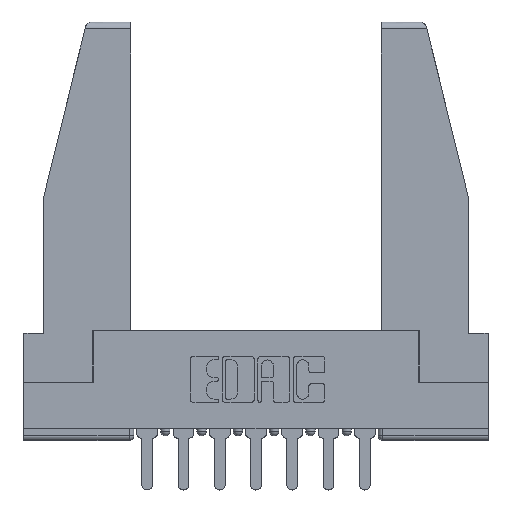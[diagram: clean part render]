
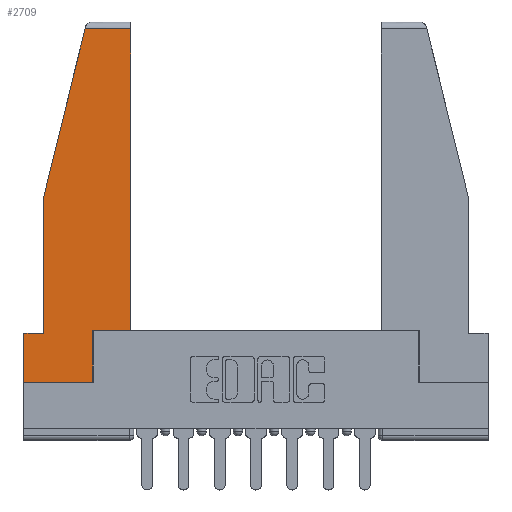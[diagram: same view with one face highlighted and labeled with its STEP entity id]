
A CAD part, top view. The second image highlights one B-rep face of the part: STEP entity #2709.
In plain terms, the highlighted planar face has unit normal (0, 0, 1).
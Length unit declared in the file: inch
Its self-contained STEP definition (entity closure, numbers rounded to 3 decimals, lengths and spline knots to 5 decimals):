
#159 = DIRECTION ( 'NONE',  ( 1., 0., 0. ) ) ;
#207 = VERTEX_POINT ( 'NONE', #12697 ) ;
#845 = VECTOR ( 'NONE', #4236, 39.37008 ) ;
#994 = DIRECTION ( 'NONE',  ( 0., 1., 0. ) ) ;
#996 = DIRECTION ( 'NONE',  ( 0., 1., 0. ) ) ;
#1153 = VERTEX_POINT ( 'NONE', #11010 ) ;
#1228 = DIRECTION ( 'NONE',  ( 1., 0., 0. ) ) ;
#1569 = VECTOR ( 'NONE', #996, 39.37008 ) ;
#1634 = EDGE_CURVE ( 'NONE', #11251, #4211, #3159, .T. ) ;
#1662 = CARTESIAN_POINT ( 'NONE',  ( 0., 1.52, 0. ) ) ;
#1704 = CARTESIAN_POINT ( 'NONE',  ( 0.461, 0.223, 0. ) ) ;
#1830 = EDGE_CURVE ( 'NONE', #12103, #9312, #5680, .T. ) ;
#1930 = EDGE_CURVE ( 'NONE', #4211, #1153, #8738, .T. ) ;
#2596 = VERTEX_POINT ( 'NONE', #8861 ) ;
#2684 = FACE_OUTER_BOUND ( 'NONE', #5577, .T. ) ;
#2698 = ORIENTED_EDGE ( 'NONE', *, *, #1930, .T. ) ;
#2709 = ADVANCED_FACE ( 'NONE', ( #2684 ), #6160, .T. ) ;
#2890 = VECTOR ( 'NONE', #8896, 39.37008 ) ;
#3142 = ORIENTED_EDGE ( 'NONE', *, *, #4959, .T. ) ;
#3159 = LINE ( 'NONE', #6031, #1569 ) ;
#4101 = CARTESIAN_POINT ( 'NONE',  ( 0.086, 0.8, 0. ) ) ;
#4175 = CARTESIAN_POINT ( 'NONE',  ( 0.297, 0., 0. ) ) ;
#4211 = VERTEX_POINT ( 'NONE', #11756 ) ;
#4228 = CARTESIAN_POINT ( 'NONE',  ( 0., 0., 0. ) ) ;
#4236 = DIRECTION ( 'NONE',  ( 0., -1., 0. ) ) ;
#4328 = LINE ( 'NONE', #9168, #845 ) ;
#4407 = DIRECTION ( 'NONE',  ( 0., -1., 0. ) ) ;
#4565 = ORIENTED_EDGE ( 'NONE', *, *, #12896, .T. ) ;
#4702 = ORIENTED_EDGE ( 'NONE', *, *, #1634, .T. ) ;
#4740 = DIRECTION ( 'NONE',  ( -1., 0., 0. ) ) ;
#4813 = DIRECTION ( 'NONE',  ( -1., 0., 0. ) ) ;
#4959 = EDGE_CURVE ( 'NONE', #9312, #5747, #9187, .T. ) ;
#5338 = DIRECTION ( 'NONE',  ( -0.239, -0.971, 0. ) ) ;
#5577 = EDGE_LOOP ( 'NONE', ( #4702, #2698, #4565, #7141, #3142, #5642, #7435, #6879, #11157 ) ) ;
#5642 = ORIENTED_EDGE ( 'NONE', *, *, #6456, .T. ) ;
#5680 = LINE ( 'NONE', #6503, #7847 ) ;
#5747 = VERTEX_POINT ( 'NONE', #12834 ) ;
#5816 = CARTESIAN_POINT ( 'NONE',  ( 0., 0., 0. ) ) ;
#5894 = LINE ( 'NONE', #5816, #2890 ) ;
#6031 = CARTESIAN_POINT ( 'NONE',  ( 0.461, 0.223, 0. ) ) ;
#6160 = PLANE ( 'NONE',  #7338 ) ;
#6456 = EDGE_CURVE ( 'NONE', #5747, #207, #4328, .T. ) ;
#6503 = CARTESIAN_POINT ( 'NONE',  ( 0.086, 0.8, 0. ) ) ;
#6513 = EDGE_CURVE ( 'NONE', #2596, #11251, #12751, .T. ) ;
#6879 = ORIENTED_EDGE ( 'NONE', *, *, #10868, .T. ) ;
#6957 = EDGE_CURVE ( 'NONE', #207, #8160, #5894, .T. ) ;
#7118 = DIRECTION ( 'NONE',  ( 0., 0., 1. ) ) ;
#7141 = ORIENTED_EDGE ( 'NONE', *, *, #1830, .T. ) ;
#7338 = AXIS2_PLACEMENT_3D ( 'NONE', #4228, #7118, #159 ) ;
#7435 = ORIENTED_EDGE ( 'NONE', *, *, #6957, .T. ) ;
#7847 = VECTOR ( 'NONE', #4407, 39.37008 ) ;
#7999 = VECTOR ( 'NONE', #5338, 39.37008 ) ;
#8160 = VERTEX_POINT ( 'NONE', #4175 ) ;
#8314 = VECTOR ( 'NONE', #994, 39.37008 ) ;
#8559 = CARTESIAN_POINT ( 'NONE',  ( 0., 0.21, 0. ) ) ;
#8738 = LINE ( 'NONE', #1662, #10297 ) ;
#8861 = CARTESIAN_POINT ( 'NONE',  ( 0.297, 0.223, 0. ) ) ;
#8896 = DIRECTION ( 'NONE',  ( 1., 0., 0. ) ) ;
#9168 = CARTESIAN_POINT ( 'NONE',  ( 0., 0.21, 0. ) ) ;
#9187 = LINE ( 'NONE', #8559, #10745 ) ;
#9312 = VERTEX_POINT ( 'NONE', #10931 ) ;
#10297 = VECTOR ( 'NONE', #4813, 39.37008 ) ;
#10658 = LINE ( 'NONE', #12114, #8314 ) ;
#10745 = VECTOR ( 'NONE', #4740, 39.37008 ) ;
#10868 = EDGE_CURVE ( 'NONE', #8160, #2596, #10658, .T. ) ;
#10931 = CARTESIAN_POINT ( 'NONE',  ( 0.086, 0.21, 0. ) ) ;
#11010 = CARTESIAN_POINT ( 'NONE',  ( 0.2636, 1.52, 0. ) ) ;
#11157 = ORIENTED_EDGE ( 'NONE', *, *, #6513, .T. ) ;
#11167 = VECTOR ( 'NONE', #1228, 39.37008 ) ;
#11251 = VERTEX_POINT ( 'NONE', #1704 ) ;
#11756 = CARTESIAN_POINT ( 'NONE',  ( 0.461, 1.52, 0. ) ) ;
#12103 = VERTEX_POINT ( 'NONE', #4101 ) ;
#12114 = CARTESIAN_POINT ( 'NONE',  ( 0.297, 0., 0. ) ) ;
#12121 = CARTESIAN_POINT ( 'NONE',  ( 0.297, 0.223, 0. ) ) ;
#12215 = LINE ( 'NONE', #12327, #7999 ) ;
#12327 = CARTESIAN_POINT ( 'NONE',  ( 0.271, 1.55, 0. ) ) ;
#12697 = CARTESIAN_POINT ( 'NONE',  ( 0., 0., 0. ) ) ;
#12751 = LINE ( 'NONE', #12121, #11167 ) ;
#12834 = CARTESIAN_POINT ( 'NONE',  ( 0., 0.21, 0. ) ) ;
#12896 = EDGE_CURVE ( 'NONE', #1153, #12103, #12215, .T. ) ;
